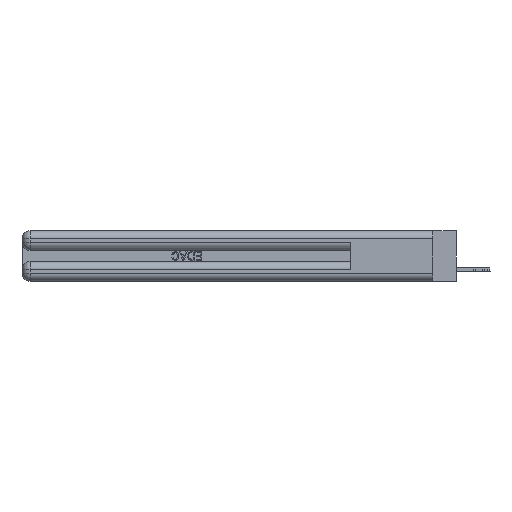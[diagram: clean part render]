
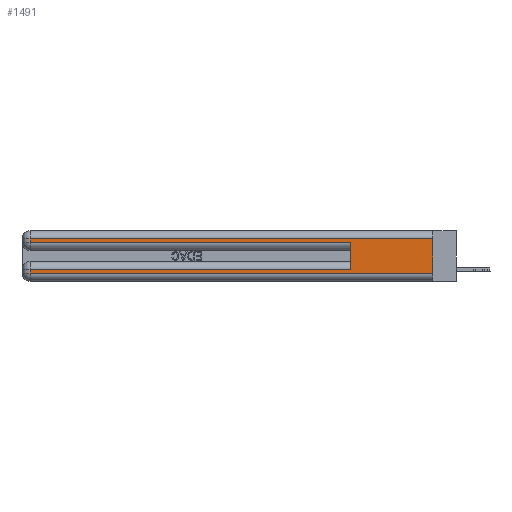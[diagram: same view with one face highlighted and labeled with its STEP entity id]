
A CAD part, left-side view. The second image highlights one B-rep face of the part: STEP entity #1491.
In plain terms, the highlighted planar face has unit normal (-1, 0, 0).
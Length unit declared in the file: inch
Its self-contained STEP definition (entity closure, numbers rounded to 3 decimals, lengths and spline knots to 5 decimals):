
#582 = LINE ( 'NONE', #20705, #49276 ) ;
#1093 = EDGE_CURVE ( 'NONE', #39350, #49088, #15531, .T. ) ;
#1491 = ADVANCED_FACE ( 'NONE', ( #23107 ), #52292, .F. ) ;
#1535 = EDGE_CURVE ( 'NONE', #41273, #31874, #11047, .T. ) ;
#1594 = DIRECTION ( 'NONE',  ( 0., 0., 1. ) ) ;
#3570 = CARTESIAN_POINT ( 'NONE',  ( 0., 2.94, 0.37 ) ) ;
#4076 = CARTESIAN_POINT ( 'NONE',  ( 0., 2.94, 0.285 ) ) ;
#5133 = CARTESIAN_POINT ( 'NONE',  ( 0., 0., 0.31 ) ) ;
#5866 = VECTOR ( 'NONE', #49852, 39.37008 ) ;
#6457 = CARTESIAN_POINT ( 'NONE',  ( 0., 2.94, 0.31 ) ) ;
#8278 = DIRECTION ( 'NONE',  ( 0., 0., -1. ) ) ;
#8562 = DIRECTION ( 'NONE',  ( 0., 0., -1. ) ) ;
#9935 = EDGE_CURVE ( 'NONE', #16331, #35400, #13053, .T. ) ;
#10017 = ORIENTED_EDGE ( 'NONE', *, *, #1535, .T. ) ;
#10266 = CARTESIAN_POINT ( 'NONE',  ( 0., 2.94, 0.37 ) ) ;
#10411 = LINE ( 'NONE', #46592, #17957 ) ;
#11047 = LINE ( 'NONE', #5133, #5866 ) ;
#12933 = VECTOR ( 'NONE', #1594, 39.37008 ) ;
#13053 = LINE ( 'NONE', #3570, #27898 ) ;
#13543 = CARTESIAN_POINT ( 'NONE',  ( 0., 2.94, 0.085 ) ) ;
#15531 = LINE ( 'NONE', #34469, #39183 ) ;
#16331 = VERTEX_POINT ( 'NONE', #13543 ) ;
#16429 = EDGE_CURVE ( 'NONE', #52639, #49088, #46153, .T. ) ;
#17607 = CARTESIAN_POINT ( 'NONE',  ( 0., 0.6, 0.145 ) ) ;
#17890 = LINE ( 'NONE', #21127, #25534 ) ;
#17957 = VECTOR ( 'NONE', #18305, 39.37008 ) ;
#18305 = DIRECTION ( 'NONE',  ( 0., 1., 0. ) ) ;
#20705 = CARTESIAN_POINT ( 'NONE',  ( 0., 0., 0.37 ) ) ;
#20885 = EDGE_CURVE ( 'NONE', #52639, #16331, #10411, .T. ) ;
#21127 = CARTESIAN_POINT ( 'NONE',  ( 0., 0., 0.06 ) ) ;
#22962 = VECTOR ( 'NONE', #26494, 39.37008 ) ;
#23107 = FACE_OUTER_BOUND ( 'NONE', #42750, .T. ) ;
#23424 = CARTESIAN_POINT ( 'NONE',  ( 0., 0., 0.37 ) ) ;
#24398 = DIRECTION ( 'NONE',  ( 0., 0., -1. ) ) ;
#24722 = EDGE_CURVE ( 'NONE', #35400, #42577, #17890, .T. ) ;
#25534 = VECTOR ( 'NONE', #47351, 39.37008 ) ;
#25566 = ORIENTED_EDGE ( 'NONE', *, *, #9935, .T. ) ;
#26494 = DIRECTION ( 'NONE',  ( 0., 0., -1. ) ) ;
#27576 = DIRECTION ( 'NONE',  ( 1., 0., 0. ) ) ;
#27898 = VECTOR ( 'NONE', #24398, 39.37008 ) ;
#30443 = ORIENTED_EDGE ( 'NONE', *, *, #16429, .F. ) ;
#31874 = VERTEX_POINT ( 'NONE', #6457 ) ;
#34469 = CARTESIAN_POINT ( 'NONE',  ( 0., 0., 0.285 ) ) ;
#34482 = ORIENTED_EDGE ( 'NONE', *, *, #46948, .F. ) ;
#35400 = VERTEX_POINT ( 'NONE', #50218 ) ;
#35823 = ORIENTED_EDGE ( 'NONE', *, *, #52876, .T. ) ;
#37960 = ORIENTED_EDGE ( 'NONE', *, *, #24722, .T. ) ;
#39183 = VECTOR ( 'NONE', #50391, 39.37008 ) ;
#39275 = AXIS2_PLACEMENT_3D ( 'NONE', #23424, #27576, #8562 ) ;
#39350 = VERTEX_POINT ( 'NONE', #4076 ) ;
#40179 = CARTESIAN_POINT ( 'NONE',  ( 0., 0., 0.31 ) ) ;
#41273 = VERTEX_POINT ( 'NONE', #40179 ) ;
#41450 = CARTESIAN_POINT ( 'NONE',  ( 0., 0.6, 0.285 ) ) ;
#42577 = VERTEX_POINT ( 'NONE', #46701 ) ;
#42750 = EDGE_LOOP ( 'NONE', ( #34482, #10017, #35823, #46693, #30443, #48377, #25566, #37960 ) ) ;
#45342 = CARTESIAN_POINT ( 'NONE',  ( 0., 0.6, 0.085 ) ) ;
#46010 = LINE ( 'NONE', #10266, #22962 ) ;
#46153 = LINE ( 'NONE', #17607, #12933 ) ;
#46592 = CARTESIAN_POINT ( 'NONE',  ( 0., 0., 0.085 ) ) ;
#46693 = ORIENTED_EDGE ( 'NONE', *, *, #1093, .T. ) ;
#46701 = CARTESIAN_POINT ( 'NONE',  ( 0., 0., 0.06 ) ) ;
#46948 = EDGE_CURVE ( 'NONE', #41273, #42577, #582, .T. ) ;
#47351 = DIRECTION ( 'NONE',  ( 0., -1., 0. ) ) ;
#48377 = ORIENTED_EDGE ( 'NONE', *, *, #20885, .T. ) ;
#49088 = VERTEX_POINT ( 'NONE', #41450 ) ;
#49276 = VECTOR ( 'NONE', #8278, 39.37008 ) ;
#49852 = DIRECTION ( 'NONE',  ( 0., 1., 0. ) ) ;
#50218 = CARTESIAN_POINT ( 'NONE',  ( 0., 2.94, 0.06 ) ) ;
#50391 = DIRECTION ( 'NONE',  ( 0., -1., 0. ) ) ;
#52292 = PLANE ( 'NONE',  #39275 ) ;
#52639 = VERTEX_POINT ( 'NONE', #45342 ) ;
#52876 = EDGE_CURVE ( 'NONE', #31874, #39350, #46010, .T. ) ;
